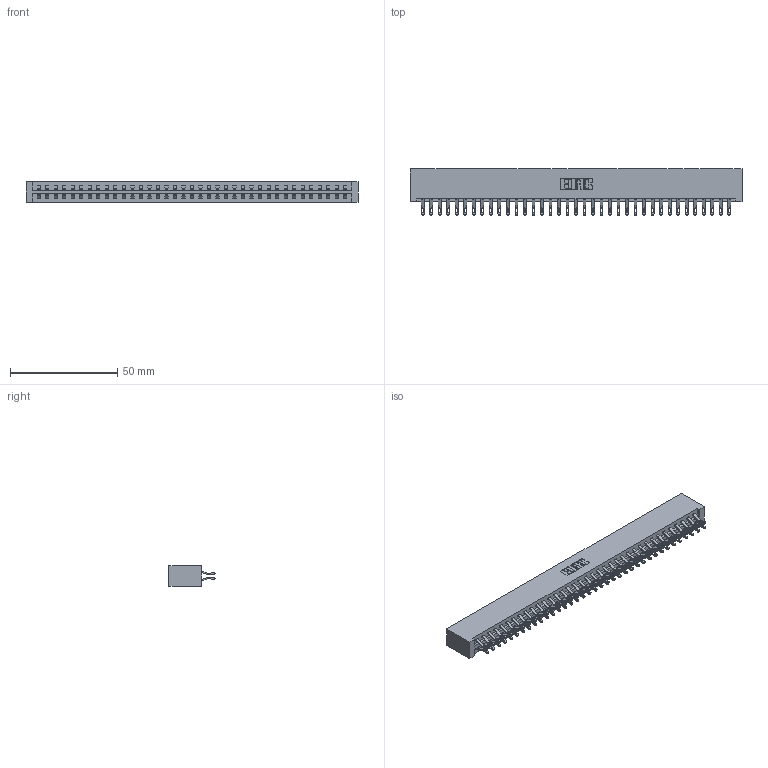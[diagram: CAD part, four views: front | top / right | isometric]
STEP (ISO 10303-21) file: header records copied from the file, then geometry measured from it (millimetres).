
FILE_DESCRIPTION (( 'STEP AP203' ), '1' );
FILE_NAME ('387-074-555-201.STEP', '2018-09-22T20:13:54', ( '' ), ( '' ), 'SwSTEP 2.0', 'SolidWorks 2016', '' );
FILE_SCHEMA (( 'CONFIG_CONTROL_DESIGN' ));
Length unit declared in the file: inch
Products named in the file (3): 337 Part_No Mounting Lugs; 345-292-001_555 Tail; 387-074-555-201
Assembly tree (75 placements, depth 2):
  387-074-555-201
    337 Part_No Mounting Lugs
    345-292-001_555 Tail  x74
Bounding box: 154.48 x 21.47 x 9.4 mm (x, y, z)
Volume: 17189.4 mm3; surface area: 20249.1 mm2
Topology: 75 solids, 75 shells, 4546 faces, 14273 edges, 9514 vertices
Faces by surface type: plane 2730, cylinder 1816
Entity records: 29383 total; most frequent: CARTESIAN_POINT 4988, ORIENTED_EDGE 4894, DIRECTION 4215, EDGE_CURVE 2447, LINE 2307, VECTOR 2307, VERTEX_POINT 1630, AXIS2_PLACEMENT_3D 954
